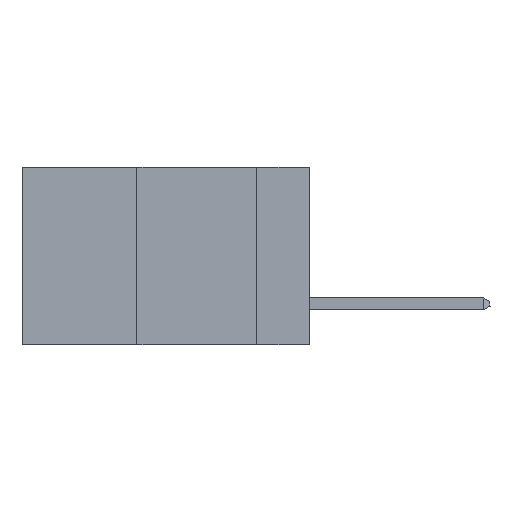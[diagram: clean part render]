
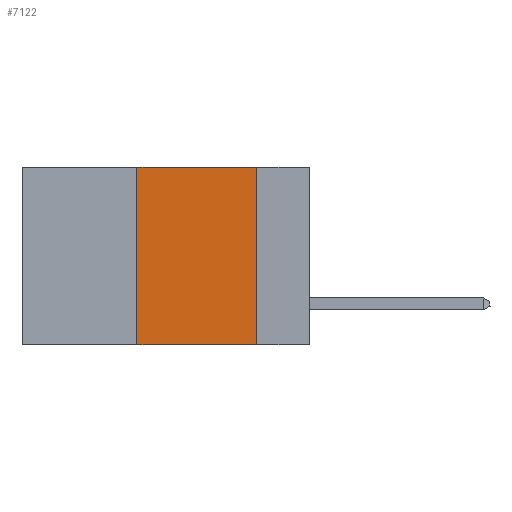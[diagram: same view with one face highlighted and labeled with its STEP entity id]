
A CAD part, left-side view. The second image highlights one B-rep face of the part: STEP entity #7122.
In plain terms, the highlighted planar face has unit normal (-1, 0, 0).
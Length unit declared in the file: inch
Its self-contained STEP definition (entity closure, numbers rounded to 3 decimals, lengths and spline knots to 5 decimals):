
#983 = EDGE_CURVE ( 'NONE', #38271, #6268, #9383, .T. ) ;
#3090 = CARTESIAN_POINT ( 'NONE',  ( 0., 0.36, 0. ) ) ;
#3659 = LINE ( 'NONE', #33946, #18504 ) ;
#6268 = VERTEX_POINT ( 'NONE', #16537 ) ;
#6615 = VERTEX_POINT ( 'NONE', #10397 ) ;
#7122 = ADVANCED_FACE ( 'NONE', ( #19521 ), #36438, .F. ) ;
#9383 = LINE ( 'NONE', #22552, #35804 ) ;
#10397 = CARTESIAN_POINT ( 'NONE',  ( 0., 0.11, -0.37 ) ) ;
#10550 = LINE ( 'NONE', #32418, #23532 ) ;
#11663 = EDGE_CURVE ( 'NONE', #30429, #6615, #10550, .T. ) ;
#12623 = EDGE_CURVE ( 'NONE', #30429, #38271, #30614, .T. ) ;
#13103 = EDGE_LOOP ( 'NONE', ( #26736, #23340, #23150, #19894 ) ) ;
#16537 = CARTESIAN_POINT ( 'NONE',  ( 0., 0.11, 0. ) ) ;
#17759 = DIRECTION ( 'NONE',  ( 0., -1., 0. ) ) ;
#18504 = VECTOR ( 'NONE', #37016, 39.37008 ) ;
#19521 = FACE_OUTER_BOUND ( 'NONE', #13103, .T. ) ;
#19591 = DIRECTION ( 'NONE',  ( 0., -1., 0. ) ) ;
#19894 = ORIENTED_EDGE ( 'NONE', *, *, #11663, .T. ) ;
#20904 = CARTESIAN_POINT ( 'NONE',  ( 0., 0.6, 0. ) ) ;
#21777 = DIRECTION ( 'NONE',  ( 0., 0., 1. ) ) ;
#22441 = VECTOR ( 'NONE', #21777, 39.37008 ) ;
#22552 = CARTESIAN_POINT ( 'NONE',  ( 0., 0.6, 0. ) ) ;
#23150 = ORIENTED_EDGE ( 'NONE', *, *, #12623, .F. ) ;
#23340 = ORIENTED_EDGE ( 'NONE', *, *, #983, .F. ) ;
#23532 = VECTOR ( 'NONE', #17759, 39.37008 ) ;
#23610 = DIRECTION ( 'NONE',  ( 0., 0., -1. ) ) ;
#26736 = ORIENTED_EDGE ( 'NONE', *, *, #27339, .F. ) ;
#27339 = EDGE_CURVE ( 'NONE', #6268, #6615, #3659, .T. ) ;
#28777 = CARTESIAN_POINT ( 'NONE',  ( 0., 0.36, 0. ) ) ;
#30429 = VERTEX_POINT ( 'NONE', #39361 ) ;
#30614 = LINE ( 'NONE', #3090, #22441 ) ;
#32418 = CARTESIAN_POINT ( 'NONE',  ( 0., 0.6, -0.37 ) ) ;
#33946 = CARTESIAN_POINT ( 'NONE',  ( 0., 0.11, 0. ) ) ;
#35804 = VECTOR ( 'NONE', #19591, 39.37008 ) ;
#35914 = DIRECTION ( 'NONE',  ( 1., 0., 0. ) ) ;
#36438 = PLANE ( 'NONE',  #39474 ) ;
#37016 = DIRECTION ( 'NONE',  ( 0., 0., -1. ) ) ;
#38271 = VERTEX_POINT ( 'NONE', #28777 ) ;
#39361 = CARTESIAN_POINT ( 'NONE',  ( 0., 0.36, -0.37 ) ) ;
#39474 = AXIS2_PLACEMENT_3D ( 'NONE', #20904, #35914, #23610 ) ;
